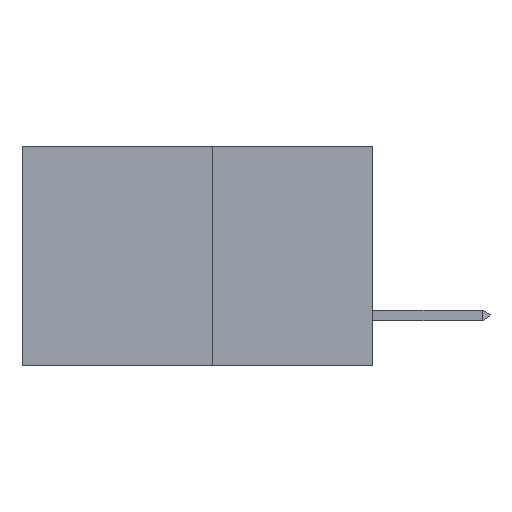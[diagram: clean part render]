
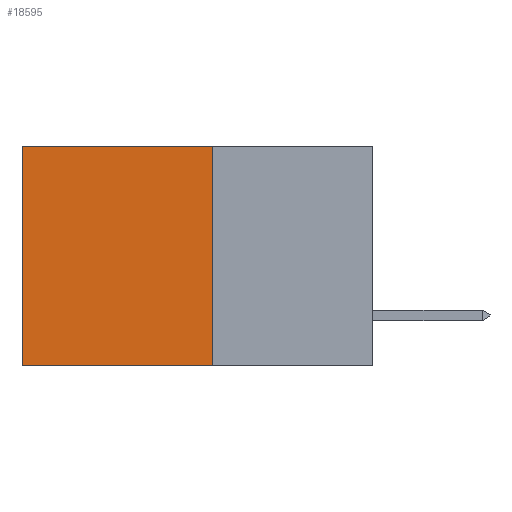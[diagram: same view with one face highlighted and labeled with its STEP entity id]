
A CAD part, left-side view. The second image highlights one B-rep face of the part: STEP entity #18595.
In plain terms, the highlighted planar face has unit normal (-1, 0, 0).
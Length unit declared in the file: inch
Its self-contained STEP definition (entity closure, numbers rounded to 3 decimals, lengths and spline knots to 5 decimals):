
#447 = VECTOR ( 'NONE', #15287, 39.37008 ) ;
#749 = VECTOR ( 'NONE', #19785, 39.37008 ) ;
#873 = VERTEX_POINT ( 'NONE', #13047 ) ;
#1445 = EDGE_LOOP ( 'NONE', ( #2730, #13112, #2482, #2810 ) ) ;
#1758 = DIRECTION ( 'NONE',  ( 0., 1., 0. ) ) ;
#2001 = CARTESIAN_POINT ( 'NONE',  ( 0.277, 0.27, -0.37 ) ) ;
#2482 = ORIENTED_EDGE ( 'NONE', *, *, #2756, .F. ) ;
#2730 = ORIENTED_EDGE ( 'NONE', *, *, #17925, .T. ) ;
#2756 = EDGE_CURVE ( 'NONE', #10577, #11497, #19699, .T. ) ;
#2810 = ORIENTED_EDGE ( 'NONE', *, *, #14699, .T. ) ;
#3431 = DIRECTION ( 'NONE',  ( 0., 0., -1. ) ) ;
#4963 = CARTESIAN_POINT ( 'NONE',  ( 0.277, 0.27, 0. ) ) ;
#5202 = LINE ( 'NONE', #4963, #749 ) ;
#6941 = EDGE_CURVE ( 'NONE', #11497, #10402, #8617, .T. ) ;
#8617 = LINE ( 'NONE', #2001, #21177 ) ;
#8769 = CARTESIAN_POINT ( 'NONE',  ( 0.277, 0.27, -0.37 ) ) ;
#10381 = DIRECTION ( 'NONE',  ( 0., 0., -1. ) ) ;
#10402 = VERTEX_POINT ( 'NONE', #18297 ) ;
#10577 = VERTEX_POINT ( 'NONE', #17120 ) ;
#11497 = VERTEX_POINT ( 'NONE', #17756 ) ;
#11827 = CARTESIAN_POINT ( 'NONE',  ( 0.277, 0.27, -0.37 ) ) ;
#13047 = CARTESIAN_POINT ( 'NONE',  ( 0.277, 0.59, 0. ) ) ;
#13112 = ORIENTED_EDGE ( 'NONE', *, *, #6941, .F. ) ;
#13688 = AXIS2_PLACEMENT_3D ( 'NONE', #8769, #20239, #10381 ) ;
#14699 = EDGE_CURVE ( 'NONE', #10577, #873, #5202, .T. ) ;
#15287 = DIRECTION ( 'NONE',  ( 0., 0., -1. ) ) ;
#15317 = VECTOR ( 'NONE', #3431, 39.37008 ) ;
#16882 = CARTESIAN_POINT ( 'NONE',  ( 0.277, 0.59, -0.37 ) ) ;
#16924 = PLANE ( 'NONE',  #13688 ) ;
#17120 = CARTESIAN_POINT ( 'NONE',  ( 0.277, 0.27, 0. ) ) ;
#17699 = FACE_OUTER_BOUND ( 'NONE', #1445, .T. ) ;
#17756 = CARTESIAN_POINT ( 'NONE',  ( 0.277, 0.27, -0.37 ) ) ;
#17925 = EDGE_CURVE ( 'NONE', #873, #10402, #17993, .T. ) ;
#17993 = LINE ( 'NONE', #16882, #447 ) ;
#18297 = CARTESIAN_POINT ( 'NONE',  ( 0.277, 0.59, -0.37 ) ) ;
#18595 = ADVANCED_FACE ( 'NONE', ( #17699 ), #16924, .F. ) ;
#19699 = LINE ( 'NONE', #11827, #15317 ) ;
#19785 = DIRECTION ( 'NONE',  ( 0., 1., 0. ) ) ;
#20239 = DIRECTION ( 'NONE',  ( 1., 0., 0. ) ) ;
#21177 = VECTOR ( 'NONE', #1758, 39.37008 ) ;
